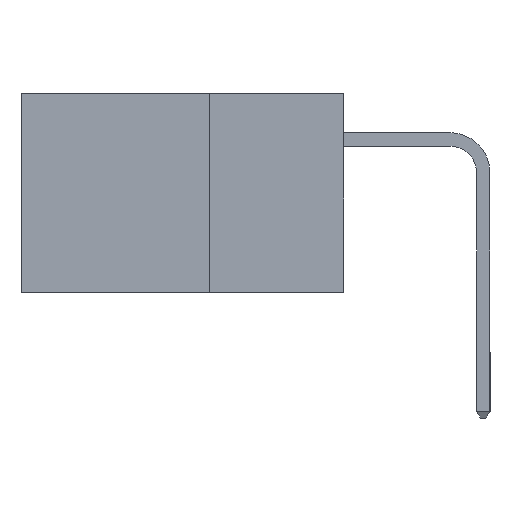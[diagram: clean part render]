
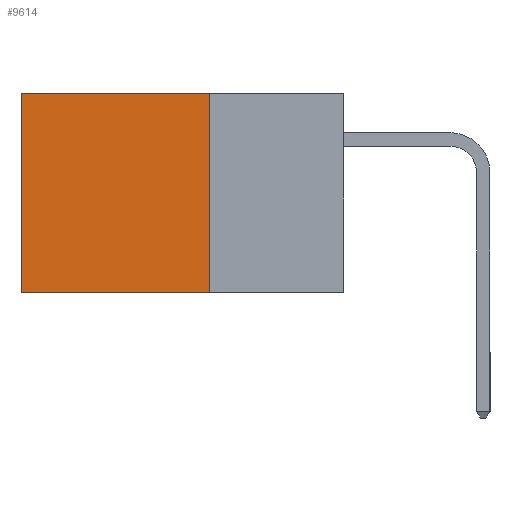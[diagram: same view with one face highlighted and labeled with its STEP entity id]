
A CAD part, left-side view. The second image highlights one B-rep face of the part: STEP entity #9614.
In plain terms, the highlighted planar face has unit normal (-1, 0, 0).
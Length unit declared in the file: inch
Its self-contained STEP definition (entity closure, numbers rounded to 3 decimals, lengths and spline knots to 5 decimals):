
#17 = ORIENTED_EDGE ( 'NONE', *, *, #780, .F. ) ;
#150 = EDGE_LOOP ( 'NONE', ( #12103, #17, #1672, #8543 ) ) ;
#780 = EDGE_CURVE ( 'NONE', #15145, #12232, #13156, .T. ) ;
#1028 = LINE ( 'NONE', #13693, #17130 ) ;
#1672 = ORIENTED_EDGE ( 'NONE', *, *, #8720, .F. ) ;
#1833 = FACE_OUTER_BOUND ( 'NONE', #150, .T. ) ;
#2690 = VECTOR ( 'NONE', #18103, 39.37008 ) ;
#3513 = CARTESIAN_POINT ( 'NONE',  ( 0.2615, 0.25, -0.37 ) ) ;
#3950 = EDGE_CURVE ( 'NONE', #13789, #12232, #10693, .T. ) ;
#5056 = DIRECTION ( 'NONE',  ( 1., 0., 0. ) ) ;
#5701 = CARTESIAN_POINT ( 'NONE',  ( 0.2615, 0.6, -0.37 ) ) ;
#5887 = CARTESIAN_POINT ( 'NONE',  ( 0.2615, 0.25, -0.37 ) ) ;
#7380 = AXIS2_PLACEMENT_3D ( 'NONE', #3513, #5056, #14316 ) ;
#8543 = ORIENTED_EDGE ( 'NONE', *, *, #19184, .T. ) ;
#8720 = EDGE_CURVE ( 'NONE', #13552, #15145, #16651, .T. ) ;
#8777 = CARTESIAN_POINT ( 'NONE',  ( 0.2615, 0.25, -0.37 ) ) ;
#8898 = DIRECTION ( 'NONE',  ( 0., 1., 0. ) ) ;
#9184 = DIRECTION ( 'NONE',  ( 0., 0., -1. ) ) ;
#9614 = ADVANCED_FACE ( 'NONE', ( #1833 ), #17700, .F. ) ;
#10693 = LINE ( 'NONE', #5701, #18183 ) ;
#12103 = ORIENTED_EDGE ( 'NONE', *, *, #3950, .T. ) ;
#12232 = VERTEX_POINT ( 'NONE', #20425 ) ;
#13156 = LINE ( 'NONE', #19850, #2690 ) ;
#13188 = CARTESIAN_POINT ( 'NONE',  ( 0.2615, 0.25, 0. ) ) ;
#13552 = VERTEX_POINT ( 'NONE', #13188 ) ;
#13693 = CARTESIAN_POINT ( 'NONE',  ( 0.2615, 0.25, 0. ) ) ;
#13789 = VERTEX_POINT ( 'NONE', #19783 ) ;
#14316 = DIRECTION ( 'NONE',  ( 0., 0., -1. ) ) ;
#15145 = VERTEX_POINT ( 'NONE', #5887 ) ;
#15298 = VECTOR ( 'NONE', #9184, 39.37008 ) ;
#15469 = DIRECTION ( 'NONE',  ( 0., 0., -1. ) ) ;
#16651 = LINE ( 'NONE', #8777, #15298 ) ;
#17130 = VECTOR ( 'NONE', #8898, 39.37008 ) ;
#17700 = PLANE ( 'NONE',  #7380 ) ;
#18103 = DIRECTION ( 'NONE',  ( 0., 1., 0. ) ) ;
#18183 = VECTOR ( 'NONE', #15469, 39.37008 ) ;
#19184 = EDGE_CURVE ( 'NONE', #13552, #13789, #1028, .T. ) ;
#19783 = CARTESIAN_POINT ( 'NONE',  ( 0.2615, 0.6, 0. ) ) ;
#19850 = CARTESIAN_POINT ( 'NONE',  ( 0.2615, 0.25, -0.37 ) ) ;
#20425 = CARTESIAN_POINT ( 'NONE',  ( 0.2615, 0.6, -0.37 ) ) ;
